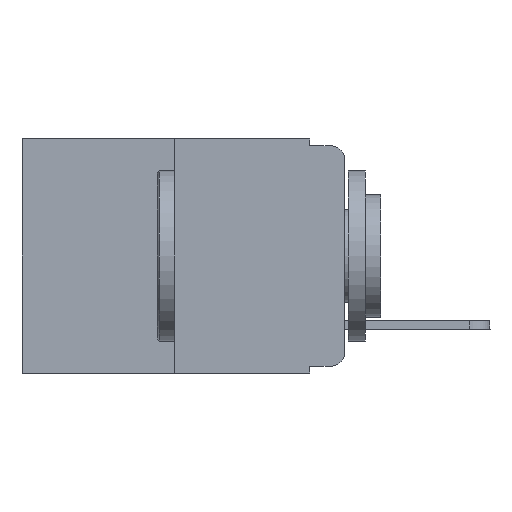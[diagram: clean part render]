
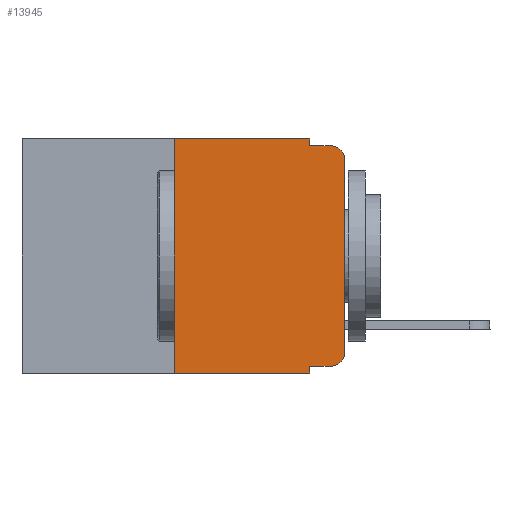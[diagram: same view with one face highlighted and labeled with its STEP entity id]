
A CAD part, left-side view. The second image highlights one B-rep face of the part: STEP entity #13945.
In plain terms, the highlighted planar face has unit normal (-1, 0, 0).
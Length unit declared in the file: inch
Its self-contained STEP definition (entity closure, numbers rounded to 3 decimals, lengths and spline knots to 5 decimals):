
#83 = VECTOR ( 'NONE', #12669, 39.37008 ) ;
#181 = PLANE ( 'NONE',  #4906 ) ;
#303 = CARTESIAN_POINT ( 'NONE',  ( 0., 0.02, -0.01 ) ) ;
#367 = ORIENTED_EDGE ( 'NONE', *, *, #14856, .T. ) ;
#865 = LINE ( 'NONE', #20305, #11048 ) ;
#1727 = VERTEX_POINT ( 'NONE', #13891 ) ;
#1761 = DIRECTION ( 'NONE',  ( 1., 0., 0. ) ) ;
#1913 = EDGE_CURVE ( 'NONE', #17573, #1727, #10138, .T. ) ;
#2348 = VECTOR ( 'NONE', #12053, 39.37008 ) ;
#2496 = DIRECTION ( 'NONE',  ( 0., 0., -1. ) ) ;
#2680 = CARTESIAN_POINT ( 'NONE',  ( 0., 0.02, -0.333 ) ) ;
#2703 = DIRECTION ( 'NONE',  ( 0., -1., 0. ) ) ;
#3162 = CARTESIAN_POINT ( 'NONE',  ( 0., 0.051, -0.343 ) ) ;
#3359 = CARTESIAN_POINT ( 'NONE',  ( 0., 0.473, 0. ) ) ;
#3658 = EDGE_CURVE ( 'NONE', #16986, #4391, #6827, .T. ) ;
#3769 = ORIENTED_EDGE ( 'NONE', *, *, #1913, .F. ) ;
#3779 = CIRCLE ( 'NONE', #4454, 0.02 ) ;
#4373 = DIRECTION ( 'NONE',  ( 0., 0., -1. ) ) ;
#4391 = VERTEX_POINT ( 'NONE', #5724 ) ;
#4454 = AXIS2_PLACEMENT_3D ( 'NONE', #17282, #9279, #14211 ) ;
#4559 = VECTOR ( 'NONE', #4373, 39.37008 ) ;
#4612 = ORIENTED_EDGE ( 'NONE', *, *, #3658, .T. ) ;
#4622 = VERTEX_POINT ( 'NONE', #303 ) ;
#4702 = VERTEX_POINT ( 'NONE', #13272 ) ;
#4840 = EDGE_CURVE ( 'NONE', #4391, #4622, #3779, .T. ) ;
#4906 = AXIS2_PLACEMENT_3D ( 'NONE', #3359, #1761, #8241 ) ;
#4911 = CARTESIAN_POINT ( 'NONE',  ( 0., 0.051, -0.333 ) ) ;
#5468 = CARTESIAN_POINT ( 'NONE',  ( 0., 0.051, 0. ) ) ;
#5724 = CARTESIAN_POINT ( 'NONE',  ( 0., 0., -0.03 ) ) ;
#5843 = DIRECTION ( 'NONE',  ( 0., 0., 1. ) ) ;
#6079 = CARTESIAN_POINT ( 'NONE',  ( 0., 0.051, 0. ) ) ;
#6267 = LINE ( 'NONE', #12544, #12072 ) ;
#6656 = EDGE_CURVE ( 'NONE', #1727, #4622, #10771, .T. ) ;
#6827 = LINE ( 'NONE', #9679, #12340 ) ;
#6950 = VERTEX_POINT ( 'NONE', #2680 ) ;
#7117 = LINE ( 'NONE', #15218, #7313 ) ;
#7313 = VECTOR ( 'NONE', #13597, 39.37008 ) ;
#7728 = ORIENTED_EDGE ( 'NONE', *, *, #20872, .F. ) ;
#8241 = DIRECTION ( 'NONE',  ( 0., 0., -1. ) ) ;
#8268 = EDGE_CURVE ( 'NONE', #8470, #10154, #20830, .T. ) ;
#8470 = VERTEX_POINT ( 'NONE', #11489 ) ;
#9279 = DIRECTION ( 'NONE',  ( -1., 0., 0. ) ) ;
#9301 = CARTESIAN_POINT ( 'NONE',  ( 0., 0., -0.313 ) ) ;
#9679 = CARTESIAN_POINT ( 'NONE',  ( 0., 0., 0. ) ) ;
#10138 = LINE ( 'NONE', #5468, #2348 ) ;
#10154 = VERTEX_POINT ( 'NONE', #3162 ) ;
#10183 = ORIENTED_EDGE ( 'NONE', *, *, #16014, .T. ) ;
#10771 = LINE ( 'NONE', #15468, #11636 ) ;
#10832 = EDGE_CURVE ( 'NONE', #6950, #16986, #16063, .T. ) ;
#11048 = VECTOR ( 'NONE', #5843, 39.37008 ) ;
#11264 = EDGE_LOOP ( 'NONE', ( #4612, #18664, #14229, #3769, #15207, #7728, #367, #17150, #10183, #17576 ) ) ;
#11489 = CARTESIAN_POINT ( 'NONE',  ( 0., 0.051, -0.333 ) ) ;
#11636 = VECTOR ( 'NONE', #2703, 39.37008 ) ;
#11977 = AXIS2_PLACEMENT_3D ( 'NONE', #13885, #17272, #2496 ) ;
#12053 = DIRECTION ( 'NONE',  ( 0., 0., -1. ) ) ;
#12072 = VECTOR ( 'NONE', #15729, 39.37008 ) ;
#12340 = VECTOR ( 'NONE', #19771, 39.37008 ) ;
#12544 = CARTESIAN_POINT ( 'NONE',  ( 0., 0.473, 0. ) ) ;
#12669 = DIRECTION ( 'NONE',  ( 0., -1., 0. ) ) ;
#12988 = LINE ( 'NONE', #4911, #83 ) ;
#13272 = CARTESIAN_POINT ( 'NONE',  ( 0., 0.25, -0.343 ) ) ;
#13597 = DIRECTION ( 'NONE',  ( 0., -1., 0. ) ) ;
#13667 = CARTESIAN_POINT ( 'NONE',  ( 0., 0.25, 0. ) ) ;
#13885 = CARTESIAN_POINT ( 'NONE',  ( 0., 0.02, -0.313 ) ) ;
#13891 = CARTESIAN_POINT ( 'NONE',  ( 0., 0.051, -0.01 ) ) ;
#13945 = ADVANCED_FACE ( 'NONE', ( #16126 ), #181, .F. ) ;
#14211 = DIRECTION ( 'NONE',  ( 0., 0., -1. ) ) ;
#14229 = ORIENTED_EDGE ( 'NONE', *, *, #6656, .F. ) ;
#14564 = EDGE_CURVE ( 'NONE', #15214, #17573, #6267, .T. ) ;
#14856 = EDGE_CURVE ( 'NONE', #4702, #10154, #7117, .T. ) ;
#15207 = ORIENTED_EDGE ( 'NONE', *, *, #14564, .F. ) ;
#15214 = VERTEX_POINT ( 'NONE', #13667 ) ;
#15218 = CARTESIAN_POINT ( 'NONE',  ( 0., 0.473, -0.343 ) ) ;
#15468 = CARTESIAN_POINT ( 'NONE',  ( 0., 0.051, -0.01 ) ) ;
#15729 = DIRECTION ( 'NONE',  ( 0., -1., 0. ) ) ;
#16014 = EDGE_CURVE ( 'NONE', #8470, #6950, #12988, .T. ) ;
#16063 = CIRCLE ( 'NONE', #11977, 0.02 ) ;
#16126 = FACE_OUTER_BOUND ( 'NONE', #11264, .T. ) ;
#16986 = VERTEX_POINT ( 'NONE', #9301 ) ;
#17150 = ORIENTED_EDGE ( 'NONE', *, *, #8268, .F. ) ;
#17272 = DIRECTION ( 'NONE',  ( -1., 0., 0. ) ) ;
#17282 = CARTESIAN_POINT ( 'NONE',  ( 0., 0.02, -0.03 ) ) ;
#17573 = VERTEX_POINT ( 'NONE', #18599 ) ;
#17576 = ORIENTED_EDGE ( 'NONE', *, *, #10832, .T. ) ;
#18599 = CARTESIAN_POINT ( 'NONE',  ( 0., 0.051, 0. ) ) ;
#18664 = ORIENTED_EDGE ( 'NONE', *, *, #4840, .T. ) ;
#19771 = DIRECTION ( 'NONE',  ( 0., 0., 1. ) ) ;
#20305 = CARTESIAN_POINT ( 'NONE',  ( 0., 0.25, 0. ) ) ;
#20830 = LINE ( 'NONE', #6079, #4559 ) ;
#20872 = EDGE_CURVE ( 'NONE', #4702, #15214, #865, .T. ) ;
